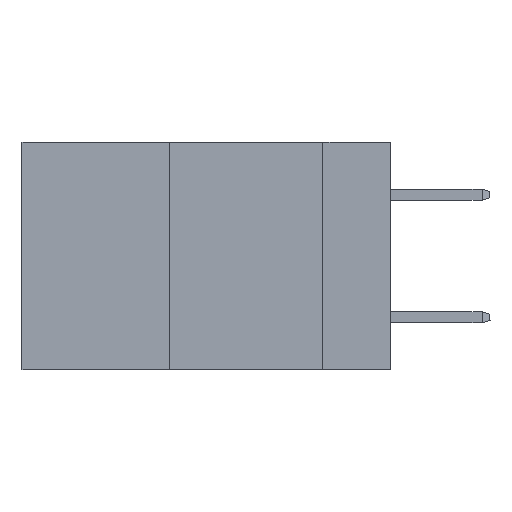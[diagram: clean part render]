
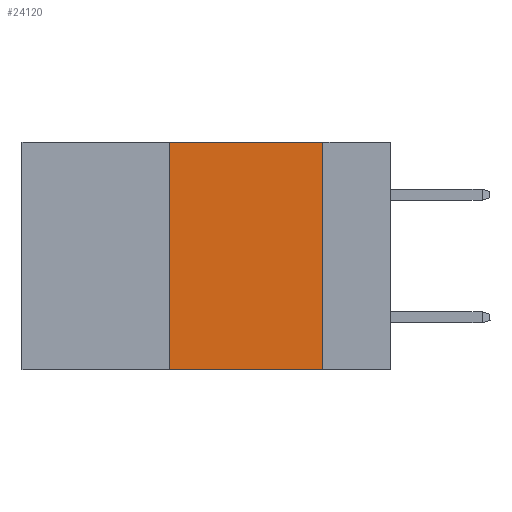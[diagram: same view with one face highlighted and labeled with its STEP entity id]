
A CAD part, left-side view. The second image highlights one B-rep face of the part: STEP entity #24120.
In plain terms, the highlighted planar face has unit normal (-1, 0, 0).
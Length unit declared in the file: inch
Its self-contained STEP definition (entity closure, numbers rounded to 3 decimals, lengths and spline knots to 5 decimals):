
#650 = DIRECTION ( 'NONE',  ( 1., 0., 0. ) ) ;
#1908 = CARTESIAN_POINT ( 'NONE',  ( 0., 0.11, 0. ) ) ;
#2683 = VECTOR ( 'NONE', #23562, 39.37008 ) ;
#2861 = ORIENTED_EDGE ( 'NONE', *, *, #18769, .F. ) ;
#3530 = VERTEX_POINT ( 'NONE', #19614 ) ;
#6209 = CARTESIAN_POINT ( 'NONE',  ( 0., 0.36, 0. ) ) ;
#6948 = ORIENTED_EDGE ( 'NONE', *, *, #18490, .F. ) ;
#7111 = LINE ( 'NONE', #6209, #20844 ) ;
#8256 = AXIS2_PLACEMENT_3D ( 'NONE', #23578, #650, #17811 ) ;
#8977 = LINE ( 'NONE', #17598, #24549 ) ;
#9291 = CARTESIAN_POINT ( 'NONE',  ( 0., 0.6, -0.37 ) ) ;
#9443 = DIRECTION ( 'NONE',  ( 0., -1., 0. ) ) ;
#9868 = VECTOR ( 'NONE', #9443, 39.37008 ) ;
#9976 = VERTEX_POINT ( 'NONE', #12603 ) ;
#10563 = ORIENTED_EDGE ( 'NONE', *, *, #12486, .F. ) ;
#12020 = ORIENTED_EDGE ( 'NONE', *, *, #16537, .T. ) ;
#12415 = DIRECTION ( 'NONE',  ( 0., -1., 0. ) ) ;
#12486 = EDGE_CURVE ( 'NONE', #23630, #3530, #7111, .T. ) ;
#12603 = CARTESIAN_POINT ( 'NONE',  ( 0., 0.11, -0.37 ) ) ;
#14379 = LINE ( 'NONE', #9291, #9868 ) ;
#14603 = CARTESIAN_POINT ( 'NONE',  ( 0., 0.36, -0.37 ) ) ;
#15490 = EDGE_LOOP ( 'NONE', ( #2861, #6948, #10563, #12020 ) ) ;
#16537 = EDGE_CURVE ( 'NONE', #23630, #9976, #14379, .T. ) ;
#17598 = CARTESIAN_POINT ( 'NONE',  ( 0., 0.6, 0. ) ) ;
#17811 = DIRECTION ( 'NONE',  ( 0., 0., -1. ) ) ;
#18490 = EDGE_CURVE ( 'NONE', #3530, #21359, #8977, .T. ) ;
#18769 = EDGE_CURVE ( 'NONE', #21359, #9976, #19696, .T. ) ;
#19614 = CARTESIAN_POINT ( 'NONE',  ( 0., 0.36, 0. ) ) ;
#19696 = LINE ( 'NONE', #23645, #2683 ) ;
#20649 = FACE_OUTER_BOUND ( 'NONE', #15490, .T. ) ;
#20844 = VECTOR ( 'NONE', #23218, 39.37008 ) ;
#21359 = VERTEX_POINT ( 'NONE', #1908 ) ;
#21565 = PLANE ( 'NONE',  #8256 ) ;
#23218 = DIRECTION ( 'NONE',  ( 0., 0., 1. ) ) ;
#23562 = DIRECTION ( 'NONE',  ( 0., 0., -1. ) ) ;
#23578 = CARTESIAN_POINT ( 'NONE',  ( 0., 0.6, 0. ) ) ;
#23630 = VERTEX_POINT ( 'NONE', #14603 ) ;
#23645 = CARTESIAN_POINT ( 'NONE',  ( 0., 0.11, 0. ) ) ;
#24120 = ADVANCED_FACE ( 'NONE', ( #20649 ), #21565, .F. ) ;
#24549 = VECTOR ( 'NONE', #12415, 39.37008 ) ;
